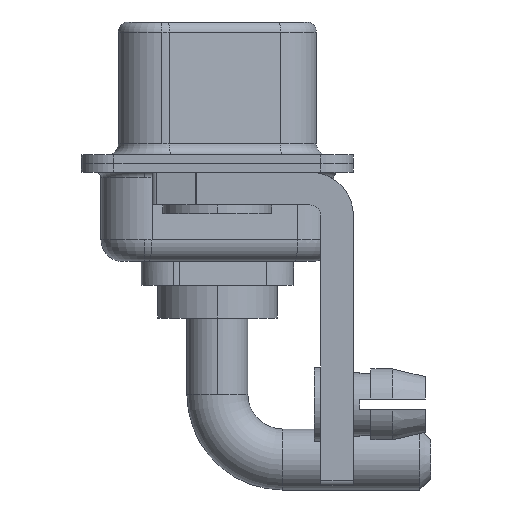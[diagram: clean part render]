
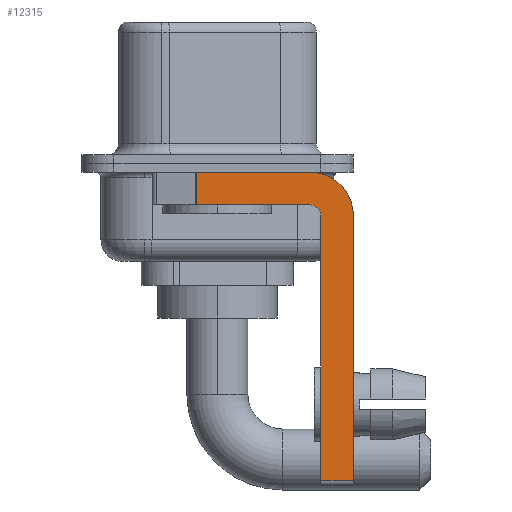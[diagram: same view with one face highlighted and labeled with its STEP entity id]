
A CAD part, left-side view. The second image highlights one B-rep face of the part: STEP entity #12315.
In plain terms, the highlighted planar face has unit normal (-1, 0, 0).
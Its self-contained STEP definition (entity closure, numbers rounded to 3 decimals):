
#660 = VERTEX_POINT ( 'NONE', #17153 ) ;
#768 = DIRECTION ( 'NONE',  ( 0., -1., 0. ) ) ;
#1434 = ORIENTED_EDGE ( 'NONE', *, *, #14871, .F. ) ;
#1798 = CARTESIAN_POINT ( 'NONE',  ( -2.9, 0.978, -1.9 ) ) ;
#2001 = CIRCLE ( 'NONE', #17199, 0.5 ) ;
#2171 = VERTEX_POINT ( 'NONE', #6289 ) ;
#2442 = LINE ( 'NONE', #5069, #15049 ) ;
#3244 = LINE ( 'NONE', #1798, #8923 ) ;
#3498 = CARTESIAN_POINT ( 'NONE',  ( -2.9, -4.75, -14.55 ) ) ;
#3702 = DIRECTION ( 'NONE',  ( 0., 0., -1. ) ) ;
#3727 = DIRECTION ( 'NONE',  ( -1., 0., 0. ) ) ;
#4784 = CARTESIAN_POINT ( 'NONE',  ( -2.9, -4.75, -14.8 ) ) ;
#5069 = CARTESIAN_POINT ( 'NONE',  ( -2.9, -4.25, -1.9 ) ) ;
#5492 = LINE ( 'NONE', #8169, #9365 ) ;
#6041 = LINE ( 'NONE', #13282, #10147 ) ;
#6079 = AXIS2_PLACEMENT_3D ( 'NONE', #14774, #10673, #10863 ) ;
#6289 = CARTESIAN_POINT ( 'NONE',  ( -2.9, -4.25, -1.9 ) ) ;
#6449 = EDGE_LOOP ( 'NONE', ( #1434, #17029, #8956, #8908, #8977, #16399, #8693, #6527 ) ) ;
#6527 = ORIENTED_EDGE ( 'NONE', *, *, #14317, .F. ) ;
#7035 = VERTEX_POINT ( 'NONE', #16090 ) ;
#7282 = CARTESIAN_POINT ( 'NONE',  ( -2.9, -6.25, -14.55 ) ) ;
#7439 = VERTEX_POINT ( 'NONE', #16911 ) ;
#7450 = DIRECTION ( 'NONE',  ( 0., 0., 1. ) ) ;
#7932 = CARTESIAN_POINT ( 'NONE',  ( -2.9, -6.25, -2.4 ) ) ;
#8115 = DIRECTION ( 'NONE',  ( 0., 1., 0. ) ) ;
#8168 = EDGE_CURVE ( 'NONE', #2171, #7439, #2442, .T. ) ;
#8169 = CARTESIAN_POINT ( 'NONE',  ( -2.9, 3., -0.4 ) ) ;
#8396 = LINE ( 'NONE', #8491, #10795 ) ;
#8436 = EDGE_CURVE ( 'NONE', #660, #7439, #3244, .T. ) ;
#8491 = CARTESIAN_POINT ( 'NONE',  ( -2.9, -6.25, -2.4 ) ) ;
#8693 = ORIENTED_EDGE ( 'NONE', *, *, #13347, .F. ) ;
#8908 = ORIENTED_EDGE ( 'NONE', *, *, #11737, .F. ) ;
#8923 = VECTOR ( 'NONE', #15793, 1000. ) ;
#8956 = ORIENTED_EDGE ( 'NONE', *, *, #8168, .F. ) ;
#8977 = ORIENTED_EDGE ( 'NONE', *, *, #12082, .F. ) ;
#9226 = CARTESIAN_POINT ( 'NONE',  ( -2.9, -4.25, -2.4 ) ) ;
#9365 = VECTOR ( 'NONE', #16683, 1000. ) ;
#9833 = VERTEX_POINT ( 'NONE', #7932 ) ;
#10147 = VECTOR ( 'NONE', #768, 1000. ) ;
#10236 = EDGE_CURVE ( 'NONE', #10707, #11927, #6041, .T. ) ;
#10673 = DIRECTION ( 'NONE',  ( 1., 0., 0. ) ) ;
#10707 = VERTEX_POINT ( 'NONE', #3498 ) ;
#10795 = VECTOR ( 'NONE', #14143, 1000. ) ;
#10863 = DIRECTION ( 'NONE',  ( 0., 0., -1. ) ) ;
#11737 = EDGE_CURVE ( 'NONE', #13663, #2171, #2001, .T. ) ;
#11927 = VERTEX_POINT ( 'NONE', #7282 ) ;
#11947 = CARTESIAN_POINT ( 'NONE',  ( -2.9, -4.25, -2.4 ) ) ;
#12082 = EDGE_CURVE ( 'NONE', #10707, #13663, #15878, .T. ) ;
#12267 = AXIS2_PLACEMENT_3D ( 'NONE', #11947, #17712, #3702 ) ;
#12315 = ADVANCED_FACE ( 'NONE', ( #16341 ), #15145, .F. ) ;
#13282 = CARTESIAN_POINT ( 'NONE',  ( -2.9, -4.25, -14.55 ) ) ;
#13347 = EDGE_CURVE ( 'NONE', #9833, #11927, #8396, .T. ) ;
#13501 = CARTESIAN_POINT ( 'NONE',  ( -2.9, -4.75, -2.4 ) ) ;
#13517 = DIRECTION ( 'NONE',  ( 0., 0., 1. ) ) ;
#13663 = VERTEX_POINT ( 'NONE', #13501 ) ;
#14143 = DIRECTION ( 'NONE',  ( 0., 0., -1. ) ) ;
#14317 = EDGE_CURVE ( 'NONE', #7035, #9833, #15483, .T. ) ;
#14774 = CARTESIAN_POINT ( 'NONE',  ( -2.9, -4.25, -2.4 ) ) ;
#14871 = EDGE_CURVE ( 'NONE', #660, #7035, #5492, .T. ) ;
#15049 = VECTOR ( 'NONE', #8115, 1000. ) ;
#15145 = PLANE ( 'NONE',  #6079 ) ;
#15483 = CIRCLE ( 'NONE', #12267, 2. ) ;
#15793 = DIRECTION ( 'NONE',  ( 0., 0., -1. ) ) ;
#15878 = LINE ( 'NONE', #4784, #16644 ) ;
#16090 = CARTESIAN_POINT ( 'NONE',  ( -2.9, -4.25, -0.4 ) ) ;
#16341 = FACE_OUTER_BOUND ( 'NONE', #6449, .T. ) ;
#16399 = ORIENTED_EDGE ( 'NONE', *, *, #10236, .T. ) ;
#16644 = VECTOR ( 'NONE', #7450, 1000. ) ;
#16683 = DIRECTION ( 'NONE',  ( 0., -1., 0. ) ) ;
#16911 = CARTESIAN_POINT ( 'NONE',  ( -2.9, 0.978, -1.9 ) ) ;
#17029 = ORIENTED_EDGE ( 'NONE', *, *, #8436, .T. ) ;
#17153 = CARTESIAN_POINT ( 'NONE',  ( -2.9, 0.978, -0.4 ) ) ;
#17199 = AXIS2_PLACEMENT_3D ( 'NONE', #9226, #3727, #13517 ) ;
#17712 = DIRECTION ( 'NONE',  ( 1., 0., 0. ) ) ;
